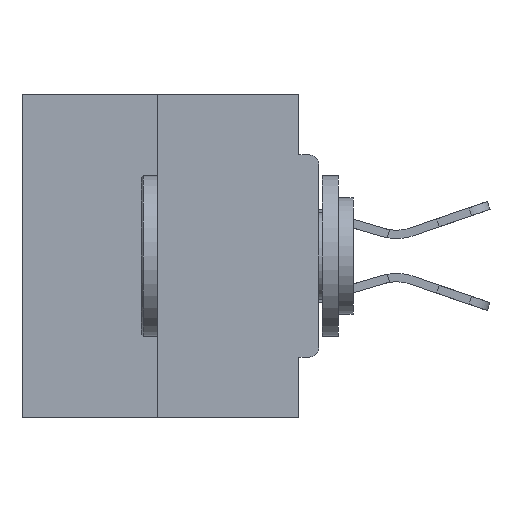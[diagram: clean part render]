
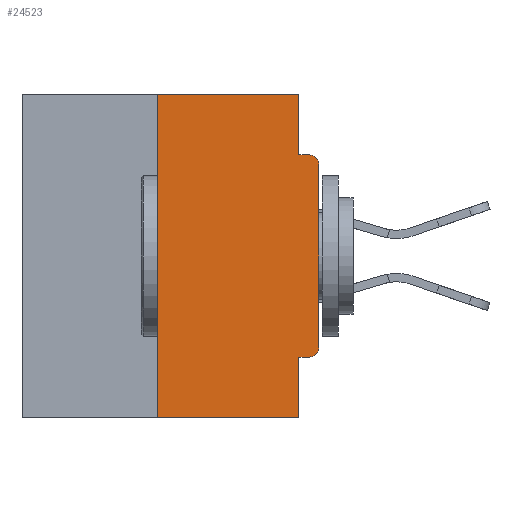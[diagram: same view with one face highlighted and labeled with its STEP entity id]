
A CAD part, left-side view. The second image highlights one B-rep face of the part: STEP entity #24523.
In plain terms, the highlighted planar face has unit normal (-1, 0, 0).
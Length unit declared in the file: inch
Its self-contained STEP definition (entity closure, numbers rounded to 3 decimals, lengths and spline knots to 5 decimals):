
#1358 = PLANE ( 'NONE',  #42174 ) ;
#1517 = CARTESIAN_POINT ( 'NONE',  ( 0., 0.25, 0. ) ) ;
#2014 = DIRECTION ( 'NONE',  ( 0., 0., -1. ) ) ;
#2471 = ORIENTED_EDGE ( 'NONE', *, *, #12608, .F. ) ;
#3299 = CARTESIAN_POINT ( 'NONE',  ( 0., 0.031, -0.5 ) ) ;
#3410 = LINE ( 'NONE', #1517, #9575 ) ;
#3475 = ORIENTED_EDGE ( 'NONE', *, *, #3530, .T. ) ;
#3530 = EDGE_CURVE ( 'NONE', #29204, #45259, #32701, .T. ) ;
#4942 = DIRECTION ( 'NONE',  ( 1., 0., 0. ) ) ;
#5102 = DIRECTION ( 'NONE',  ( 0., 0., 1. ) ) ;
#5398 = EDGE_LOOP ( 'NONE', ( #5728, #16763, #19532, #2471, #25907, #3475, #42354, #39000, #43640, #18432 ) ) ;
#5624 = EDGE_CURVE ( 'NONE', #13016, #39916, #36206, .T. ) ;
#5728 = ORIENTED_EDGE ( 'NONE', *, *, #42549, .F. ) ;
#6214 = VERTEX_POINT ( 'NONE', #18760 ) ;
#6675 = EDGE_CURVE ( 'NONE', #45259, #8978, #16725, .T. ) ;
#6705 = FACE_OUTER_BOUND ( 'NONE', #5398, .T. ) ;
#6787 = VECTOR ( 'NONE', #41573, 39.37008 ) ;
#8064 = DIRECTION ( 'NONE',  ( 0., -1., 0. ) ) ;
#8978 = VERTEX_POINT ( 'NONE', #29900 ) ;
#9575 = VECTOR ( 'NONE', #5102, 39.37008 ) ;
#10339 = LINE ( 'NONE', #41924, #30974 ) ;
#11528 = EDGE_CURVE ( 'NONE', #29204, #6214, #23802, .T. ) ;
#11844 = CARTESIAN_POINT ( 'NONE',  ( 0., 0.031, -0.0935 ) ) ;
#12608 = EDGE_CURVE ( 'NONE', #6214, #39916, #21387, .T. ) ;
#13016 = VERTEX_POINT ( 'NONE', #13489 ) ;
#13343 = DIRECTION ( 'NONE',  ( 0., 1., 0. ) ) ;
#13489 = CARTESIAN_POINT ( 'NONE',  ( 0., 0.25, -0.5 ) ) ;
#14553 = DIRECTION ( 'NONE',  ( 0., 0., -1. ) ) ;
#14734 = CARTESIAN_POINT ( 'NONE',  ( 0., 0.25, 0. ) ) ;
#16725 = LINE ( 'NONE', #24317, #38404 ) ;
#16763 = ORIENTED_EDGE ( 'NONE', *, *, #23480, .F. ) ;
#18432 = ORIENTED_EDGE ( 'NONE', *, *, #21043, .F. ) ;
#18760 = CARTESIAN_POINT ( 'NONE',  ( 0., 0.031, -0.4065 ) ) ;
#19484 = CARTESIAN_POINT ( 'NONE',  ( 0., 0.46, 0. ) ) ;
#19532 = ORIENTED_EDGE ( 'NONE', *, *, #5624, .T. ) ;
#19907 = VECTOR ( 'NONE', #31986, 39.37008 ) ;
#20091 = CIRCLE ( 'NONE', #44853, 0.015 ) ;
#21043 = EDGE_CURVE ( 'NONE', #31712, #32521, #31044, .T. ) ;
#21387 = LINE ( 'NONE', #30389, #45323 ) ;
#21916 = CARTESIAN_POINT ( 'NONE',  ( 0., 0.46, -0.5 ) ) ;
#22060 = AXIS2_PLACEMENT_3D ( 'NONE', #37479, #44178, #37167 ) ;
#23480 = EDGE_CURVE ( 'NONE', #13016, #33843, #3410, .T. ) ;
#23709 = CARTESIAN_POINT ( 'NONE',  ( 0., 0., -0.3915 ) ) ;
#23802 = LINE ( 'NONE', #33281, #41560 ) ;
#24317 = CARTESIAN_POINT ( 'NONE',  ( 0., 0., 0. ) ) ;
#24523 = ADVANCED_FACE ( 'NONE', ( #6705 ), #1358, .F. ) ;
#25907 = ORIENTED_EDGE ( 'NONE', *, *, #11528, .F. ) ;
#25947 = CARTESIAN_POINT ( 'NONE',  ( 0., 0.031, 0. ) ) ;
#26833 = CARTESIAN_POINT ( 'NONE',  ( 0., 0.015, -0.0935 ) ) ;
#28425 = VECTOR ( 'NONE', #8064, 39.37008 ) ;
#28712 = DIRECTION ( 'NONE',  ( -1., 0., 0. ) ) ;
#29204 = VERTEX_POINT ( 'NONE', #34867 ) ;
#29900 = CARTESIAN_POINT ( 'NONE',  ( 0., 0., -0.1085 ) ) ;
#30389 = CARTESIAN_POINT ( 'NONE',  ( 0., 0.031, -0.5 ) ) ;
#30673 = VERTEX_POINT ( 'NONE', #26833 ) ;
#30974 = VECTOR ( 'NONE', #45516, 39.37008 ) ;
#31044 = LINE ( 'NONE', #35274, #19907 ) ;
#31712 = VERTEX_POINT ( 'NONE', #25947 ) ;
#31986 = DIRECTION ( 'NONE',  ( 0., 0., -1. ) ) ;
#32464 = CARTESIAN_POINT ( 'NONE',  ( 0., 0.015, -0.1085 ) ) ;
#32521 = VERTEX_POINT ( 'NONE', #11844 ) ;
#32701 = CIRCLE ( 'NONE', #22060, 0.015 ) ;
#33281 = CARTESIAN_POINT ( 'NONE',  ( 0., 0., -0.4065 ) ) ;
#33843 = VERTEX_POINT ( 'NONE', #14734 ) ;
#34545 = DIRECTION ( 'NONE',  ( 0., 0., 1. ) ) ;
#34867 = CARTESIAN_POINT ( 'NONE',  ( 0., 0.015, -0.4065 ) ) ;
#35274 = CARTESIAN_POINT ( 'NONE',  ( 0., 0.031, 0. ) ) ;
#36206 = LINE ( 'NONE', #21916, #28425 ) ;
#37167 = DIRECTION ( 'NONE',  ( 0., 0., -1. ) ) ;
#37479 = CARTESIAN_POINT ( 'NONE',  ( 0., 0.015, -0.3915 ) ) ;
#38404 = VECTOR ( 'NONE', #34545, 39.37008 ) ;
#39000 = ORIENTED_EDGE ( 'NONE', *, *, #45709, .T. ) ;
#39916 = VERTEX_POINT ( 'NONE', #3299 ) ;
#41313 = LINE ( 'NONE', #41431, #6787 ) ;
#41431 = CARTESIAN_POINT ( 'NONE',  ( 0., 0., -0.0935 ) ) ;
#41560 = VECTOR ( 'NONE', #13343, 39.37008 ) ;
#41573 = DIRECTION ( 'NONE',  ( 0., -1., 0. ) ) ;
#41924 = CARTESIAN_POINT ( 'NONE',  ( 0., 0.46, 0. ) ) ;
#42174 = AXIS2_PLACEMENT_3D ( 'NONE', #19484, #4942, #44195 ) ;
#42354 = ORIENTED_EDGE ( 'NONE', *, *, #6675, .T. ) ;
#42549 = EDGE_CURVE ( 'NONE', #33843, #31712, #10339, .T. ) ;
#43640 = ORIENTED_EDGE ( 'NONE', *, *, #44847, .F. ) ;
#44178 = DIRECTION ( 'NONE',  ( -1., 0., 0. ) ) ;
#44195 = DIRECTION ( 'NONE',  ( 0., 0., -1. ) ) ;
#44847 = EDGE_CURVE ( 'NONE', #32521, #30673, #41313, .T. ) ;
#44853 = AXIS2_PLACEMENT_3D ( 'NONE', #32464, #28712, #14553 ) ;
#45259 = VERTEX_POINT ( 'NONE', #23709 ) ;
#45323 = VECTOR ( 'NONE', #2014, 39.37008 ) ;
#45516 = DIRECTION ( 'NONE',  ( 0., -1., 0. ) ) ;
#45709 = EDGE_CURVE ( 'NONE', #8978, #30673, #20091, .T. ) ;
